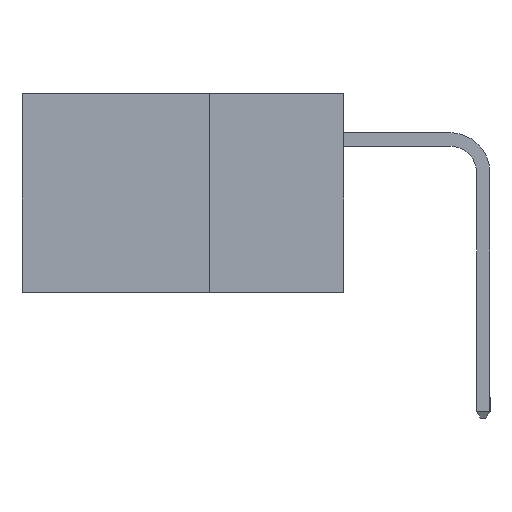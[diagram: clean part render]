
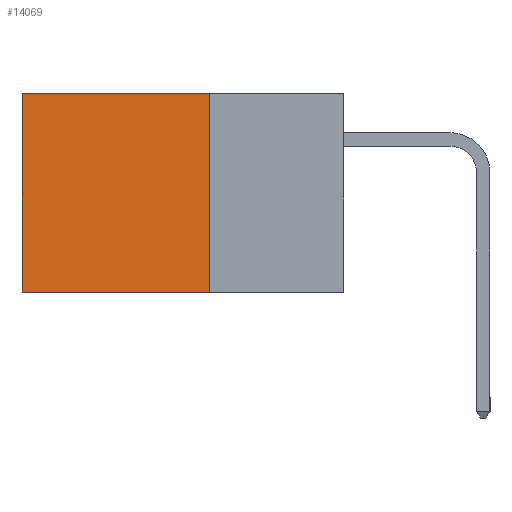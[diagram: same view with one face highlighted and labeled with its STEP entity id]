
A CAD part, left-side view. The second image highlights one B-rep face of the part: STEP entity #14069.
In plain terms, the highlighted planar face has unit normal (-1, 0, 0).
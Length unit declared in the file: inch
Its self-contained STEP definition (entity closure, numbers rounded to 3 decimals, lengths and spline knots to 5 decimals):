
#71 = CARTESIAN_POINT ( 'NONE',  ( 0.2615, 0.25, 0. ) ) ;
#444 = CARTESIAN_POINT ( 'NONE',  ( 0.2615, 0.6, -0.37 ) ) ;
#792 = EDGE_CURVE ( 'NONE', #13467, #11518, #13669, .T. ) ;
#875 = CARTESIAN_POINT ( 'NONE',  ( 0.2615, 0.25, -0.37 ) ) ;
#1548 = DIRECTION ( 'NONE',  ( 1., 0., 0. ) ) ;
#2132 = VERTEX_POINT ( 'NONE', #17450 ) ;
#3060 = DIRECTION ( 'NONE',  ( 0., 1., 0. ) ) ;
#4262 = LINE ( 'NONE', #19958, #17505 ) ;
#4745 = VERTEX_POINT ( 'NONE', #444 ) ;
#4908 = VECTOR ( 'NONE', #7669, 39.37008 ) ;
#5183 = AXIS2_PLACEMENT_3D ( 'NONE', #11803, #1548, #12772 ) ;
#5385 = LINE ( 'NONE', #14075, #4908 ) ;
#7669 = DIRECTION ( 'NONE',  ( 0., 0., -1. ) ) ;
#8098 = ORIENTED_EDGE ( 'NONE', *, *, #19879, .T. ) ;
#8188 = LINE ( 'NONE', #20433, #19766 ) ;
#8877 = ORIENTED_EDGE ( 'NONE', *, *, #13970, .T. ) ;
#9147 = EDGE_LOOP ( 'NONE', ( #8877, #18952, #17218, #8098 ) ) ;
#11518 = VERTEX_POINT ( 'NONE', #875 ) ;
#11803 = CARTESIAN_POINT ( 'NONE',  ( 0.2615, 0.25, -0.37 ) ) ;
#12112 = DIRECTION ( 'NONE',  ( 0., 1., 0. ) ) ;
#12772 = DIRECTION ( 'NONE',  ( 0., 0., -1. ) ) ;
#13467 = VERTEX_POINT ( 'NONE', #71 ) ;
#13669 = LINE ( 'NONE', #13835, #17870 ) ;
#13835 = CARTESIAN_POINT ( 'NONE',  ( 0.2615, 0.25, -0.37 ) ) ;
#13970 = EDGE_CURVE ( 'NONE', #2132, #4745, #5385, .T. ) ;
#14038 = EDGE_CURVE ( 'NONE', #11518, #4745, #8188, .T. ) ;
#14069 = ADVANCED_FACE ( 'NONE', ( #20218 ), #19002, .F. ) ;
#14075 = CARTESIAN_POINT ( 'NONE',  ( 0.2615, 0.6, -0.37 ) ) ;
#17218 = ORIENTED_EDGE ( 'NONE', *, *, #792, .F. ) ;
#17450 = CARTESIAN_POINT ( 'NONE',  ( 0.2615, 0.6, 0. ) ) ;
#17505 = VECTOR ( 'NONE', #12112, 39.37008 ) ;
#17870 = VECTOR ( 'NONE', #20291, 39.37008 ) ;
#18952 = ORIENTED_EDGE ( 'NONE', *, *, #14038, .F. ) ;
#19002 = PLANE ( 'NONE',  #5183 ) ;
#19766 = VECTOR ( 'NONE', #3060, 39.37008 ) ;
#19879 = EDGE_CURVE ( 'NONE', #13467, #2132, #4262, .T. ) ;
#19958 = CARTESIAN_POINT ( 'NONE',  ( 0.2615, 0.25, 0. ) ) ;
#20218 = FACE_OUTER_BOUND ( 'NONE', #9147, .T. ) ;
#20291 = DIRECTION ( 'NONE',  ( 0., 0., -1. ) ) ;
#20433 = CARTESIAN_POINT ( 'NONE',  ( 0.2615, 0.25, -0.37 ) ) ;
